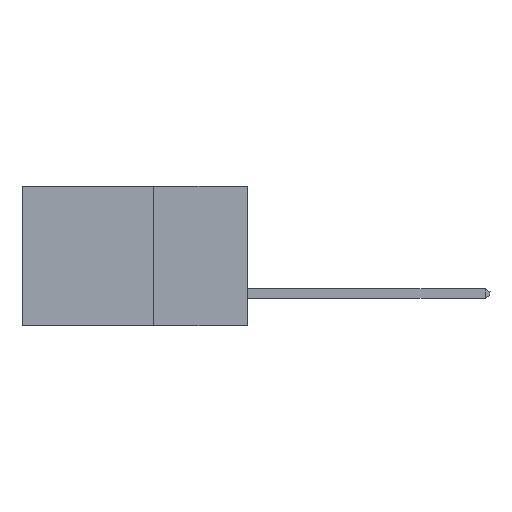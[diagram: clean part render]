
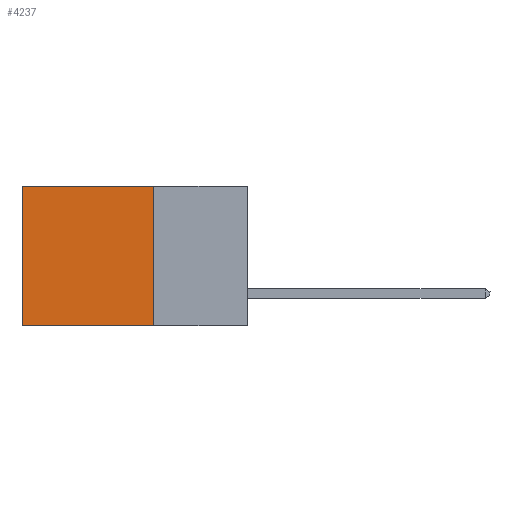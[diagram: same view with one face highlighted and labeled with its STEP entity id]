
A CAD part, left-side view. The second image highlights one B-rep face of the part: STEP entity #4237.
In plain terms, the highlighted planar face has unit normal (-1, 0, 0).
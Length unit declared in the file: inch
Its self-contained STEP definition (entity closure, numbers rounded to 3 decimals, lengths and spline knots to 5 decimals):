
#459 = CARTESIAN_POINT ( 'NONE',  ( 0.2615, 0.25, -0.37 ) ) ;
#756 = ORIENTED_EDGE ( 'NONE', *, *, #8513, .T. ) ;
#944 = VECTOR ( 'NONE', #1265, 39.37008 ) ;
#1078 = VECTOR ( 'NONE', #4972, 39.37008 ) ;
#1237 = CARTESIAN_POINT ( 'NONE',  ( 0.2615, 0.6, 0. ) ) ;
#1265 = DIRECTION ( 'NONE',  ( 0., 0., -1. ) ) ;
#1670 = VERTEX_POINT ( 'NONE', #1237 ) ;
#1887 = VERTEX_POINT ( 'NONE', #8984 ) ;
#2405 = DIRECTION ( 'NONE',  ( 1., 0., 0. ) ) ;
#2452 = CARTESIAN_POINT ( 'NONE',  ( 0.2615, 0.25, -0.37 ) ) ;
#2467 = AXIS2_PLACEMENT_3D ( 'NONE', #2452, #2405, #3860 ) ;
#2517 = EDGE_CURVE ( 'NONE', #4071, #6344, #8233, .T. ) ;
#2553 = DIRECTION ( 'NONE',  ( 0., 1., 0. ) ) ;
#2729 = CARTESIAN_POINT ( 'NONE',  ( 0.2615, 0.6, -0.37 ) ) ;
#2833 = VECTOR ( 'NONE', #2553, 39.37008 ) ;
#3068 = EDGE_CURVE ( 'NONE', #1670, #6344, #8512, .T. ) ;
#3300 = FACE_OUTER_BOUND ( 'NONE', #3729, .T. ) ;
#3398 = CARTESIAN_POINT ( 'NONE',  ( 0.2615, 0.25, 0. ) ) ;
#3729 = EDGE_LOOP ( 'NONE', ( #6848, #4765, #8150, #756 ) ) ;
#3860 = DIRECTION ( 'NONE',  ( 0., 0., -1. ) ) ;
#4071 = VERTEX_POINT ( 'NONE', #6582 ) ;
#4134 = LINE ( 'NONE', #3398, #1078 ) ;
#4237 = ADVANCED_FACE ( 'NONE', ( #3300 ), #7476, .F. ) ;
#4646 = CARTESIAN_POINT ( 'NONE',  ( 0.2615, 0.25, -0.37 ) ) ;
#4765 = ORIENTED_EDGE ( 'NONE', *, *, #2517, .F. ) ;
#4814 = CARTESIAN_POINT ( 'NONE',  ( 0.2615, 0.6, -0.37 ) ) ;
#4815 = EDGE_CURVE ( 'NONE', #1887, #4071, #5529, .T. ) ;
#4930 = VECTOR ( 'NONE', #5622, 39.37008 ) ;
#4972 = DIRECTION ( 'NONE',  ( 0., 1., 0. ) ) ;
#5529 = LINE ( 'NONE', #459, #4930 ) ;
#5622 = DIRECTION ( 'NONE',  ( 0., 0., -1. ) ) ;
#6344 = VERTEX_POINT ( 'NONE', #4814 ) ;
#6582 = CARTESIAN_POINT ( 'NONE',  ( 0.2615, 0.25, -0.37 ) ) ;
#6848 = ORIENTED_EDGE ( 'NONE', *, *, #3068, .T. ) ;
#7476 = PLANE ( 'NONE',  #2467 ) ;
#8150 = ORIENTED_EDGE ( 'NONE', *, *, #4815, .F. ) ;
#8233 = LINE ( 'NONE', #4646, #2833 ) ;
#8512 = LINE ( 'NONE', #2729, #944 ) ;
#8513 = EDGE_CURVE ( 'NONE', #1887, #1670, #4134, .T. ) ;
#8984 = CARTESIAN_POINT ( 'NONE',  ( 0.2615, 0.25, 0. ) ) ;
